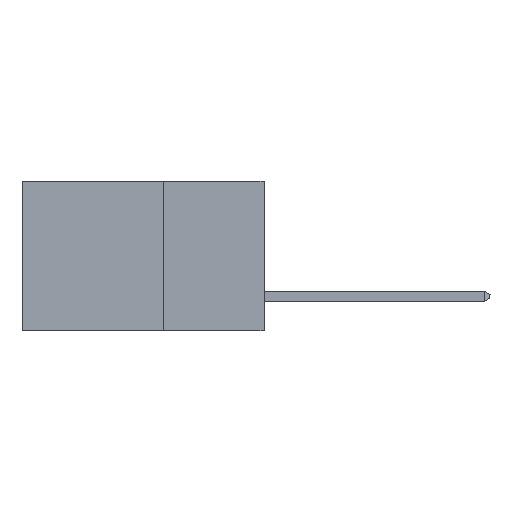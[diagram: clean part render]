
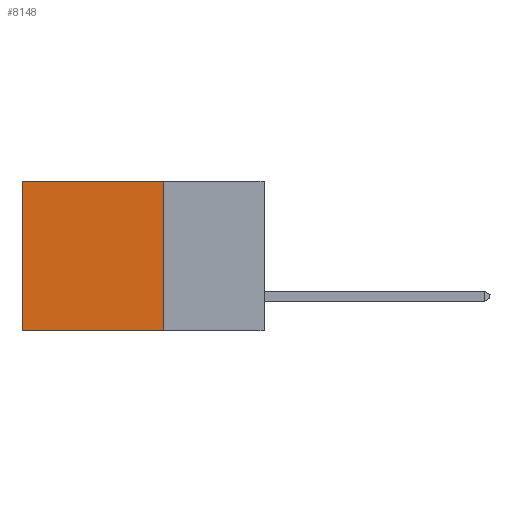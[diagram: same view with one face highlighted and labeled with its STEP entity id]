
A CAD part, left-side view. The second image highlights one B-rep face of the part: STEP entity #8148.
In plain terms, the highlighted planar face has unit normal (-1, 0, 0).
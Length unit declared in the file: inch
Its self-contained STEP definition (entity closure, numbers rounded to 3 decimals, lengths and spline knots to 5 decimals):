
#595 = DIRECTION ( 'NONE',  ( 0., 0., -1. ) ) ;
#756 = ORIENTED_EDGE ( 'NONE', *, *, #12764, .F. ) ;
#1145 = LINE ( 'NONE', #10374, #12797 ) ;
#2028 = VERTEX_POINT ( 'NONE', #3795 ) ;
#2220 = DIRECTION ( 'NONE',  ( 0., 1., 0. ) ) ;
#2285 = LINE ( 'NONE', #8561, #8180 ) ;
#3196 = VECTOR ( 'NONE', #8653, 39.37008 ) ;
#3524 = FACE_OUTER_BOUND ( 'NONE', #8978, .T. ) ;
#3715 = AXIS2_PLACEMENT_3D ( 'NONE', #6596, #10718, #595 ) ;
#3795 = CARTESIAN_POINT ( 'NONE',  ( 0.2615, 0.6, -0.37 ) ) ;
#4002 = CARTESIAN_POINT ( 'NONE',  ( 0.2615, 0.25, 0. ) ) ;
#4433 = CARTESIAN_POINT ( 'NONE',  ( 0.2615, 0.6, 0. ) ) ;
#5215 = DIRECTION ( 'NONE',  ( 0., 0., -1. ) ) ;
#5354 = DIRECTION ( 'NONE',  ( 0., 1., 0. ) ) ;
#6318 = ORIENTED_EDGE ( 'NONE', *, *, #11687, .T. ) ;
#6324 = CARTESIAN_POINT ( 'NONE',  ( 0.2615, 0.25, -0.37 ) ) ;
#6596 = CARTESIAN_POINT ( 'NONE',  ( 0.2615, 0.25, -0.37 ) ) ;
#8148 = ADVANCED_FACE ( 'NONE', ( #3524 ), #12879, .F. ) ;
#8180 = VECTOR ( 'NONE', #5354, 39.37008 ) ;
#8486 = EDGE_CURVE ( 'NONE', #9964, #9370, #1145, .T. ) ;
#8561 = CARTESIAN_POINT ( 'NONE',  ( 0.2615, 0.25, -0.37 ) ) ;
#8653 = DIRECTION ( 'NONE',  ( 0., 0., -1. ) ) ;
#8978 = EDGE_LOOP ( 'NONE', ( #6318, #11305, #756, #10143 ) ) ;
#9370 = VERTEX_POINT ( 'NONE', #4433 ) ;
#9964 = VERTEX_POINT ( 'NONE', #4002 ) ;
#10143 = ORIENTED_EDGE ( 'NONE', *, *, #8486, .T. ) ;
#10161 = EDGE_CURVE ( 'NONE', #11307, #2028, #2285, .T. ) ;
#10360 = LINE ( 'NONE', #11434, #12293 ) ;
#10374 = CARTESIAN_POINT ( 'NONE',  ( 0.2615, 0.25, 0. ) ) ;
#10528 = CARTESIAN_POINT ( 'NONE',  ( 0.2615, 0.25, -0.37 ) ) ;
#10718 = DIRECTION ( 'NONE',  ( 1., 0., 0. ) ) ;
#11305 = ORIENTED_EDGE ( 'NONE', *, *, #10161, .F. ) ;
#11307 = VERTEX_POINT ( 'NONE', #6324 ) ;
#11434 = CARTESIAN_POINT ( 'NONE',  ( 0.2615, 0.6, -0.37 ) ) ;
#11687 = EDGE_CURVE ( 'NONE', #9370, #2028, #10360, .T. ) ;
#12293 = VECTOR ( 'NONE', #5215, 39.37008 ) ;
#12759 = LINE ( 'NONE', #10528, #3196 ) ;
#12764 = EDGE_CURVE ( 'NONE', #9964, #11307, #12759, .T. ) ;
#12797 = VECTOR ( 'NONE', #2220, 39.37008 ) ;
#12879 = PLANE ( 'NONE',  #3715 ) ;
